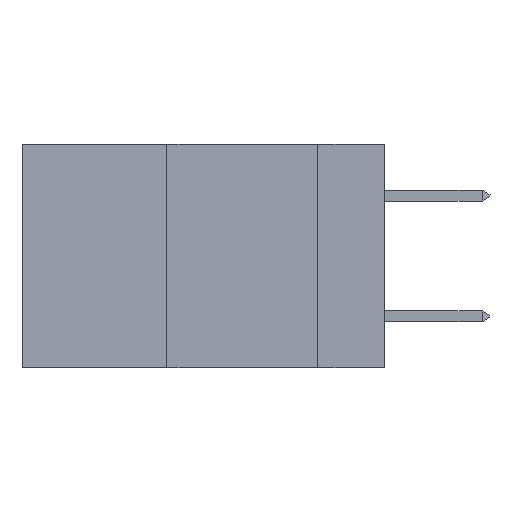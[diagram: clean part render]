
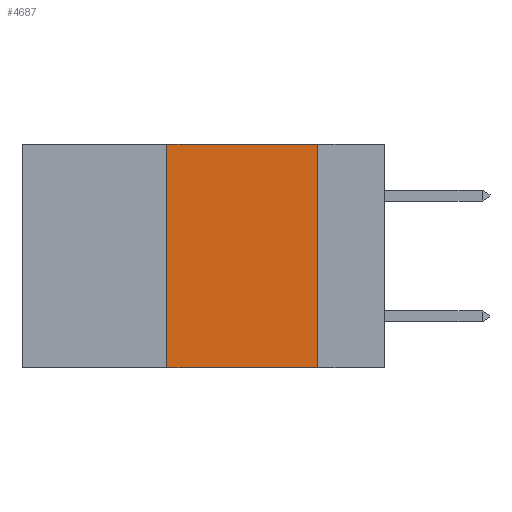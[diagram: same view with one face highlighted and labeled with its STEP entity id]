
A CAD part, left-side view. The second image highlights one B-rep face of the part: STEP entity #4687.
In plain terms, the highlighted planar face has unit normal (-1, 0, 0).
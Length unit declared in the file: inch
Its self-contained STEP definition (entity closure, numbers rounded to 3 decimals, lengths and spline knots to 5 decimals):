
#617 = DIRECTION ( 'NONE',  ( 1., 0., 0. ) ) ;
#1106 = ORIENTED_EDGE ( 'NONE', *, *, #5343, .F. ) ;
#1158 = CARTESIAN_POINT ( 'NONE',  ( 0., 0.6, 0. ) ) ;
#1601 = CARTESIAN_POINT ( 'NONE',  ( 0., 0.36, 0. ) ) ;
#1739 = LINE ( 'NONE', #9161, #11102 ) ;
#2194 = AXIS2_PLACEMENT_3D ( 'NONE', #5538, #617, #9224 ) ;
#2473 = EDGE_CURVE ( 'NONE', #12490, #2790, #7428, .T. ) ;
#2486 = DIRECTION ( 'NONE',  ( 0., 0., 1. ) ) ;
#2775 = ORIENTED_EDGE ( 'NONE', *, *, #9446, .F. ) ;
#2776 = VECTOR ( 'NONE', #2486, 39.37008 ) ;
#2790 = VERTEX_POINT ( 'NONE', #10911 ) ;
#3826 = DIRECTION ( 'NONE',  ( 0., -1., 0. ) ) ;
#3895 = ORIENTED_EDGE ( 'NONE', *, *, #2473, .F. ) ;
#4687 = ADVANCED_FACE ( 'NONE', ( #9631 ), #8016, .F. ) ;
#5263 = EDGE_LOOP ( 'NONE', ( #1106, #3895, #2775, #10157 ) ) ;
#5343 = EDGE_CURVE ( 'NONE', #2790, #13936, #1739, .T. ) ;
#5538 = CARTESIAN_POINT ( 'NONE',  ( 0., 0.6, 0. ) ) ;
#5546 = DIRECTION ( 'NONE',  ( 0., -1., 0. ) ) ;
#6481 = CARTESIAN_POINT ( 'NONE',  ( 0., 0.11, -0.37 ) ) ;
#6764 = VECTOR ( 'NONE', #3826, 39.37008 ) ;
#7428 = LINE ( 'NONE', #1158, #10266 ) ;
#7822 = CARTESIAN_POINT ( 'NONE',  ( 0., 0.36, -0.37 ) ) ;
#8016 = PLANE ( 'NONE',  #2194 ) ;
#9161 = CARTESIAN_POINT ( 'NONE',  ( 0., 0.11, 0. ) ) ;
#9224 = DIRECTION ( 'NONE',  ( 0., 0., -1. ) ) ;
#9297 = LINE ( 'NONE', #13306, #2776 ) ;
#9446 = EDGE_CURVE ( 'NONE', #9981, #12490, #9297, .T. ) ;
#9631 = FACE_OUTER_BOUND ( 'NONE', #5263, .T. ) ;
#9981 = VERTEX_POINT ( 'NONE', #7822 ) ;
#10157 = ORIENTED_EDGE ( 'NONE', *, *, #12327, .T. ) ;
#10266 = VECTOR ( 'NONE', #5546, 39.37008 ) ;
#10359 = DIRECTION ( 'NONE',  ( 0., 0., -1. ) ) ;
#10911 = CARTESIAN_POINT ( 'NONE',  ( 0., 0.11, 0. ) ) ;
#11012 = CARTESIAN_POINT ( 'NONE',  ( 0., 0.6, -0.37 ) ) ;
#11102 = VECTOR ( 'NONE', #10359, 39.37008 ) ;
#12327 = EDGE_CURVE ( 'NONE', #9981, #13936, #12737, .T. ) ;
#12490 = VERTEX_POINT ( 'NONE', #1601 ) ;
#12737 = LINE ( 'NONE', #11012, #6764 ) ;
#13306 = CARTESIAN_POINT ( 'NONE',  ( 0., 0.36, 0. ) ) ;
#13936 = VERTEX_POINT ( 'NONE', #6481 ) ;
